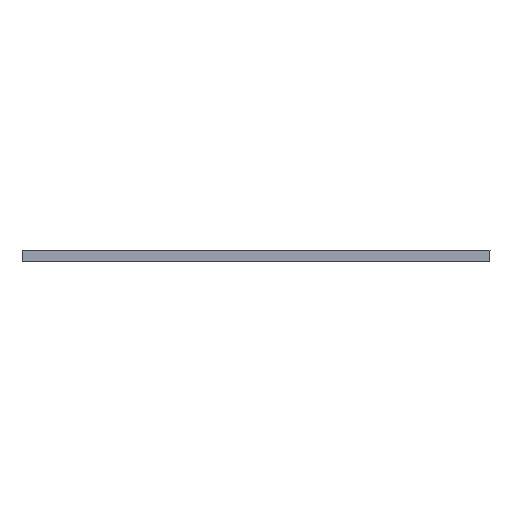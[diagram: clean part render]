
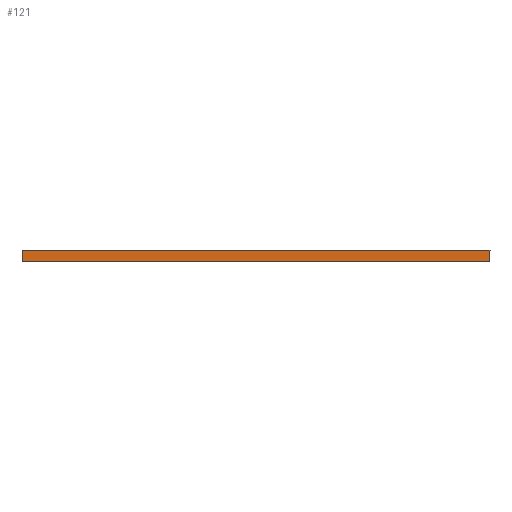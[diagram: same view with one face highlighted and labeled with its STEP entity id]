
A CAD part, left-side view. The second image highlights one B-rep face of the part: STEP entity #121.
In plain terms, the highlighted planar face has unit normal (-1, 0, 0).
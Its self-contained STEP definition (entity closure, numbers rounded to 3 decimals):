
#33 = CARTESIAN_POINT ( 'NONE',  ( -22.811, 20.5, 21.127 ) ) ;
#58 = CARTESIAN_POINT ( 'NONE',  ( -22.811, 20.5, 22.127 ) ) ;
#63 = FACE_OUTER_BOUND ( 'NONE', #1593, .T. ) ;
#90 = CARTESIAN_POINT ( 'NONE',  ( -22.811, -19.5, 22.127 ) ) ;
#104 = DIRECTION ( 'NONE',  ( 0., 0., -1. ) ) ;
#121 = ADVANCED_FACE ( 'NONE', ( #63 ), #4043, .F. ) ;
#126 = CARTESIAN_POINT ( 'NONE',  ( -22.811, 20.5, 22.127 ) ) ;
#211 = VECTOR ( 'NONE', #4622, 1000. ) ;
#433 = DIRECTION ( 'NONE',  ( 1., 0., 0. ) ) ;
#442 = LINE ( 'NONE', #126, #2386 ) ;
#1479 = ORIENTED_EDGE ( 'NONE', *, *, #3589, .T. ) ;
#1593 = EDGE_LOOP ( 'NONE', ( #2350, #1972, #4482, #1479 ) ) ;
#1906 = VERTEX_POINT ( 'NONE', #2756 ) ;
#1944 = VERTEX_POINT ( 'NONE', #2624 ) ;
#1952 = CARTESIAN_POINT ( 'NONE',  ( -22.811, 20.5, 22.127 ) ) ;
#1972 = ORIENTED_EDGE ( 'NONE', *, *, #3625, .F. ) ;
#1993 = CARTESIAN_POINT ( 'NONE',  ( -22.811, 20.5, 21.127 ) ) ;
#2011 = AXIS2_PLACEMENT_3D ( 'NONE', #58, #433, #4046 ) ;
#2066 = VERTEX_POINT ( 'NONE', #1993 ) ;
#2092 = VERTEX_POINT ( 'NONE', #1952 ) ;
#2104 = VECTOR ( 'NONE', #3861, 1000. ) ;
#2350 = ORIENTED_EDGE ( 'NONE', *, *, #3615, .T. ) ;
#2386 = VECTOR ( 'NONE', #104, 1000. ) ;
#2624 = CARTESIAN_POINT ( 'NONE',  ( -22.811, -19.5, 21.127 ) ) ;
#2756 = CARTESIAN_POINT ( 'NONE',  ( -22.811, -19.5, 22.127 ) ) ;
#3250 = VECTOR ( 'NONE', #3516, 1000. ) ;
#3381 = LINE ( 'NONE', #90, #2104 ) ;
#3516 = DIRECTION ( 'NONE',  ( 0., -1., 0. ) ) ;
#3522 = LINE ( 'NONE', #33, #211 ) ;
#3589 = EDGE_CURVE ( 'NONE', #2092, #2066, #442, .T. ) ;
#3615 = EDGE_CURVE ( 'NONE', #2066, #1944, #3522, .T. ) ;
#3625 = EDGE_CURVE ( 'NONE', #1906, #1944, #3381, .T. ) ;
#3626 = EDGE_CURVE ( 'NONE', #2092, #1906, #4248, .T. ) ;
#3861 = DIRECTION ( 'NONE',  ( 0., 0., -1. ) ) ;
#3892 = CARTESIAN_POINT ( 'NONE',  ( -22.811, 20.5, 22.127 ) ) ;
#4043 = PLANE ( 'NONE',  #2011 ) ;
#4046 = DIRECTION ( 'NONE',  ( 0., 1., 0. ) ) ;
#4248 = LINE ( 'NONE', #3892, #3250 ) ;
#4482 = ORIENTED_EDGE ( 'NONE', *, *, #3626, .F. ) ;
#4622 = DIRECTION ( 'NONE',  ( 0., -1., 0. ) ) ;
